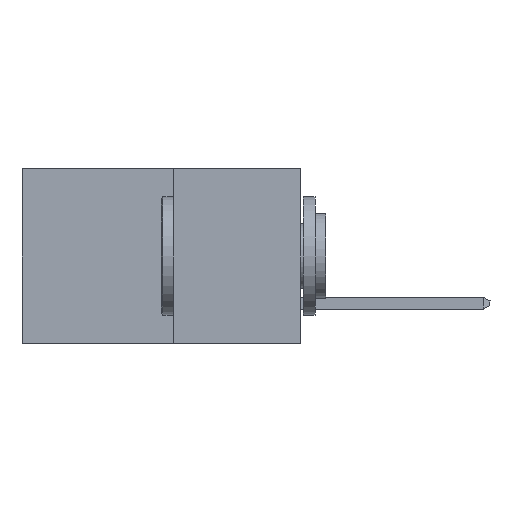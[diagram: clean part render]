
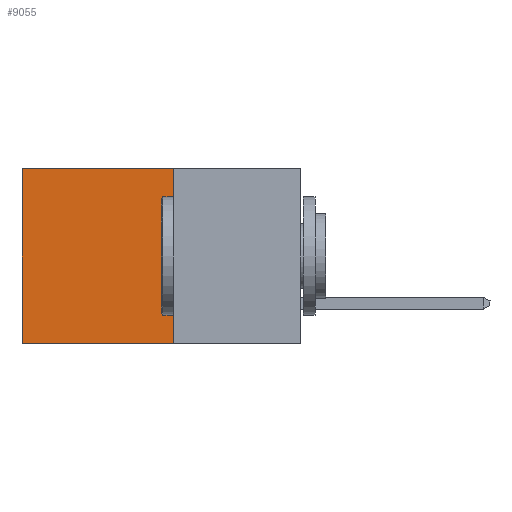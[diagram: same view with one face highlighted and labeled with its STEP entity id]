
A CAD part, left-side view. The second image highlights one B-rep face of the part: STEP entity #9055.
In plain terms, the highlighted planar face has unit normal (-1, 0, 0).
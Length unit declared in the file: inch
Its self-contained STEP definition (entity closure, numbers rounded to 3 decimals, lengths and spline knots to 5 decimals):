
#177 = CARTESIAN_POINT ( 'NONE',  ( 0.277, 0.27, -0.37 ) ) ;
#255 = EDGE_CURVE ( 'NONE', #4873, #7647, #1418, .T. ) ;
#317 = CARTESIAN_POINT ( 'NONE',  ( 0.277, 0.27, -0.37 ) ) ;
#595 = ORIENTED_EDGE ( 'NONE', *, *, #9515, .F. ) ;
#836 = EDGE_LOOP ( 'NONE', ( #2444, #8500, #595, #4805 ) ) ;
#949 = FACE_OUTER_BOUND ( 'NONE', #836, .T. ) ;
#1076 = DIRECTION ( 'NONE',  ( 0., 0., -1. ) ) ;
#1185 = VERTEX_POINT ( 'NONE', #7792 ) ;
#1265 = VERTEX_POINT ( 'NONE', #5894 ) ;
#1418 = LINE ( 'NONE', #2129, #3166 ) ;
#1519 = DIRECTION ( 'NONE',  ( 0., 1., 0. ) ) ;
#2129 = CARTESIAN_POINT ( 'NONE',  ( 0.277, 0.27, 0. ) ) ;
#2295 = CARTESIAN_POINT ( 'NONE',  ( 0.277, 0.59, 0. ) ) ;
#2444 = ORIENTED_EDGE ( 'NONE', *, *, #3770, .T. ) ;
#2553 = LINE ( 'NONE', #8255, #6309 ) ;
#2813 = DIRECTION ( 'NONE',  ( 0., 1., 0. ) ) ;
#3166 = VECTOR ( 'NONE', #1519, 39.37008 ) ;
#3298 = LINE ( 'NONE', #3544, #9238 ) ;
#3544 = CARTESIAN_POINT ( 'NONE',  ( 0.277, 0.27, -0.37 ) ) ;
#3770 = EDGE_CURVE ( 'NONE', #7647, #1185, #2553, .T. ) ;
#4657 = VECTOR ( 'NONE', #5390, 39.37008 ) ;
#4780 = PLANE ( 'NONE',  #7924 ) ;
#4805 = ORIENTED_EDGE ( 'NONE', *, *, #255, .T. ) ;
#4873 = VERTEX_POINT ( 'NONE', #6937 ) ;
#5390 = DIRECTION ( 'NONE',  ( 0., 0., -1. ) ) ;
#5541 = DIRECTION ( 'NONE',  ( 1., 0., 0. ) ) ;
#5894 = CARTESIAN_POINT ( 'NONE',  ( 0.277, 0.27, -0.37 ) ) ;
#6309 = VECTOR ( 'NONE', #8222, 39.37008 ) ;
#6937 = CARTESIAN_POINT ( 'NONE',  ( 0.277, 0.27, 0. ) ) ;
#7647 = VERTEX_POINT ( 'NONE', #2295 ) ;
#7792 = CARTESIAN_POINT ( 'NONE',  ( 0.277, 0.59, -0.37 ) ) ;
#7924 = AXIS2_PLACEMENT_3D ( 'NONE', #317, #5541, #1076 ) ;
#8077 = EDGE_CURVE ( 'NONE', #1265, #1185, #3298, .T. ) ;
#8222 = DIRECTION ( 'NONE',  ( 0., 0., -1. ) ) ;
#8255 = CARTESIAN_POINT ( 'NONE',  ( 0.277, 0.59, -0.37 ) ) ;
#8500 = ORIENTED_EDGE ( 'NONE', *, *, #8077, .F. ) ;
#8623 = LINE ( 'NONE', #177, #4657 ) ;
#9055 = ADVANCED_FACE ( 'NONE', ( #949 ), #4780, .F. ) ;
#9238 = VECTOR ( 'NONE', #2813, 39.37008 ) ;
#9515 = EDGE_CURVE ( 'NONE', #4873, #1265, #8623, .T. ) ;
